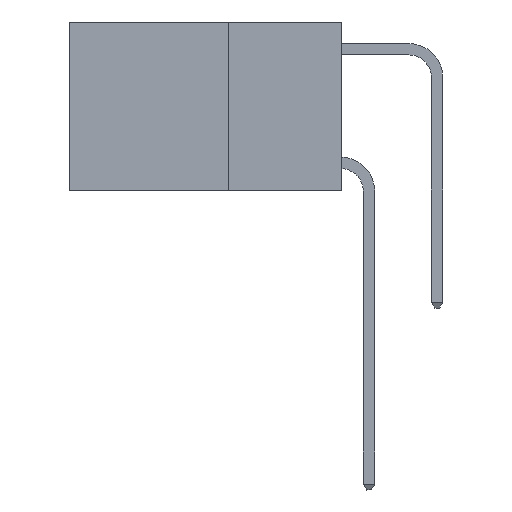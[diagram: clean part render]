
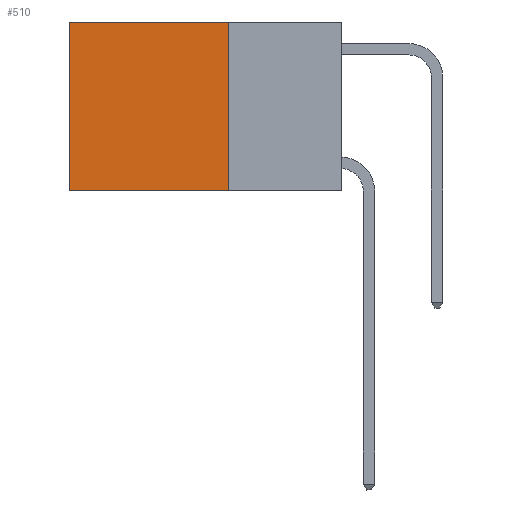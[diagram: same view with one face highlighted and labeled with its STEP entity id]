
A CAD part, left-side view. The second image highlights one B-rep face of the part: STEP entity #510.
In plain terms, the highlighted planar face has unit normal (-1, 0, 0).
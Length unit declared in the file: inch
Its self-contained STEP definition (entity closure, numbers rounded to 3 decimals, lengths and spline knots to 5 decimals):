
#181 = VECTOR ( 'NONE', #11272, 39.37008 ) ;
#510 = ADVANCED_FACE ( 'NONE', ( #10088 ), #15529, .F. ) ;
#515 = CARTESIAN_POINT ( 'NONE',  ( 0.2625, 0.25, 0. ) ) ;
#1053 = CARTESIAN_POINT ( 'NONE',  ( 0.2625, 0.25, 0. ) ) ;
#1737 = ORIENTED_EDGE ( 'NONE', *, *, #16040, .F. ) ;
#1848 = CARTESIAN_POINT ( 'NONE',  ( 0.2625, 0.6, 0. ) ) ;
#2311 = DIRECTION ( 'NONE',  ( 1., 0., 0. ) ) ;
#2805 = VECTOR ( 'NONE', #5478, 39.37008 ) ;
#3326 = EDGE_LOOP ( 'NONE', ( #6655, #1737, #10528, #10391 ) ) ;
#5478 = DIRECTION ( 'NONE',  ( 0., 0., -1. ) ) ;
#6456 = DIRECTION ( 'NONE',  ( 0., 0., -1. ) ) ;
#6545 = DIRECTION ( 'NONE',  ( 0., 0., -1. ) ) ;
#6655 = ORIENTED_EDGE ( 'NONE', *, *, #7135, .T. ) ;
#7135 = EDGE_CURVE ( 'NONE', #16152, #14599, #12191, .T. ) ;
#7166 = DIRECTION ( 'NONE',  ( 0., 1., 0. ) ) ;
#7452 = AXIS2_PLACEMENT_3D ( 'NONE', #14679, #2311, #6545 ) ;
#8554 = EDGE_CURVE ( 'NONE', #8810, #16152, #16661, .T. ) ;
#8635 = VECTOR ( 'NONE', #7166, 39.37008 ) ;
#8810 = VERTEX_POINT ( 'NONE', #1053 ) ;
#9321 = CARTESIAN_POINT ( 'NONE',  ( 0.2625, 0.25, -0.37 ) ) ;
#10088 = FACE_OUTER_BOUND ( 'NONE', #3326, .T. ) ;
#10391 = ORIENTED_EDGE ( 'NONE', *, *, #8554, .T. ) ;
#10528 = ORIENTED_EDGE ( 'NONE', *, *, #16843, .F. ) ;
#11272 = DIRECTION ( 'NONE',  ( 0., 1., 0. ) ) ;
#12191 = LINE ( 'NONE', #13339, #13214 ) ;
#13107 = LINE ( 'NONE', #15899, #2805 ) ;
#13214 = VECTOR ( 'NONE', #6456, 39.37008 ) ;
#13339 = CARTESIAN_POINT ( 'NONE',  ( 0.2625, 0.6, 0. ) ) ;
#14216 = VERTEX_POINT ( 'NONE', #9321 ) ;
#14599 = VERTEX_POINT ( 'NONE', #15844 ) ;
#14679 = CARTESIAN_POINT ( 'NONE',  ( 0.2625, 0.25, 0. ) ) ;
#15529 = PLANE ( 'NONE',  #7452 ) ;
#15844 = CARTESIAN_POINT ( 'NONE',  ( 0.2625, 0.6, -0.37 ) ) ;
#15899 = CARTESIAN_POINT ( 'NONE',  ( 0.2625, 0.25, 0. ) ) ;
#16040 = EDGE_CURVE ( 'NONE', #14216, #14599, #16561, .T. ) ;
#16152 = VERTEX_POINT ( 'NONE', #1848 ) ;
#16561 = LINE ( 'NONE', #16640, #181 ) ;
#16640 = CARTESIAN_POINT ( 'NONE',  ( 0.2625, 0.25, -0.37 ) ) ;
#16661 = LINE ( 'NONE', #515, #8635 ) ;
#16843 = EDGE_CURVE ( 'NONE', #8810, #14216, #13107, .T. ) ;
